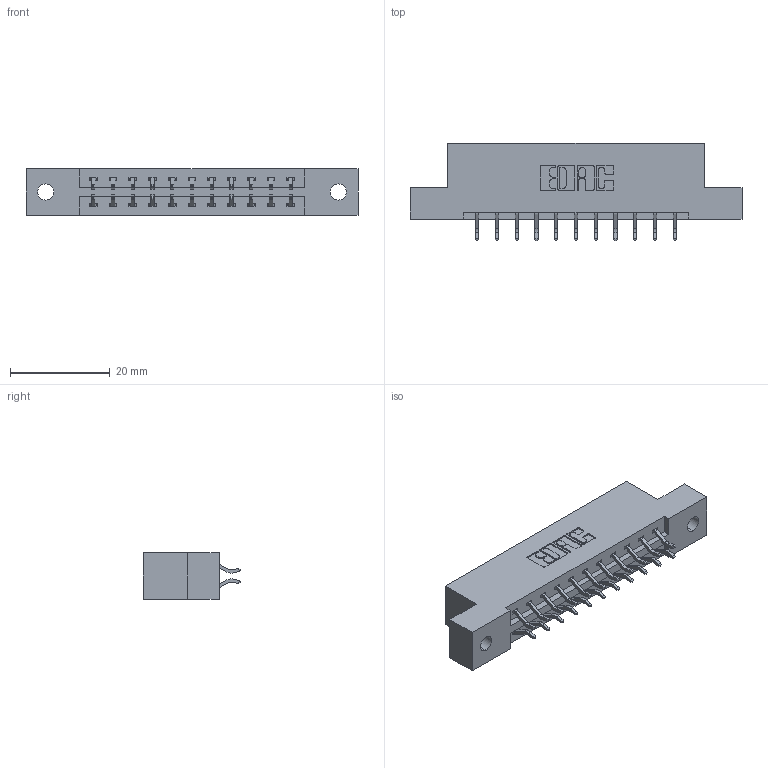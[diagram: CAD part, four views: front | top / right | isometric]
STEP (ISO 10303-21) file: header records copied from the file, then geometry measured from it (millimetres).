
FILE_DESCRIPTION (( 'STEP AP203' ), '1' );
FILE_NAME ('337-022-556-202.STEP', '2018-08-05T15:09:26', ( '' ), ( '' ), 'SwSTEP 2.0', 'SolidWorks 2016', '' );
FILE_SCHEMA (( 'CONFIG_CONTROL_DESIGN' ));
Length unit declared in the file: inch
Products named in the file (3): 337 Part_Flush Mounting Lugs - 0.128 Dia; 345-292-001_556 Tail; 337-022-556-202
Assembly tree (23 placements, depth 2):
  337-022-556-202
    337 Part_Flush Mounting Lugs - 0.128 Dia
    345-292-001_556 Tail  x22
Bounding box: 66.6 x 19.57 x 9.4 mm (x, y, z)
Volume: 6568.5 mm3; surface area: 6828.7 mm2
Topology: 23 solids, 23 shells, 1434 faces, 4249 edges, 2802 vertices
Faces by surface type: plane 994, cylinder 440
Entity records: 12761 total; most frequent: CARTESIAN_POINT 2190, ORIENTED_EDGE 2114, DIRECTION 1909, EDGE_CURVE 1057, VECTOR 921, LINE 921, VERTEX_POINT 702, AXIS2_PLACEMENT_3D 494
